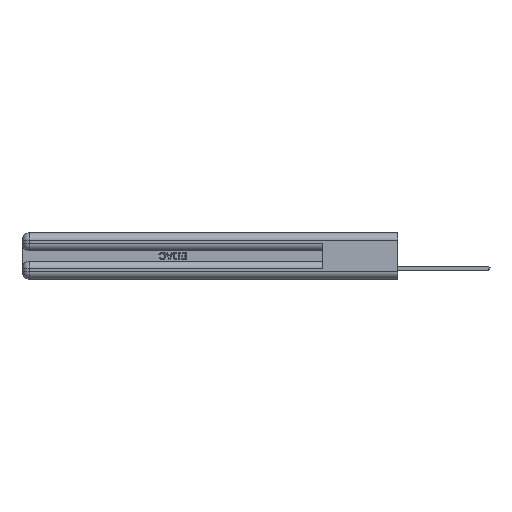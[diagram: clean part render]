
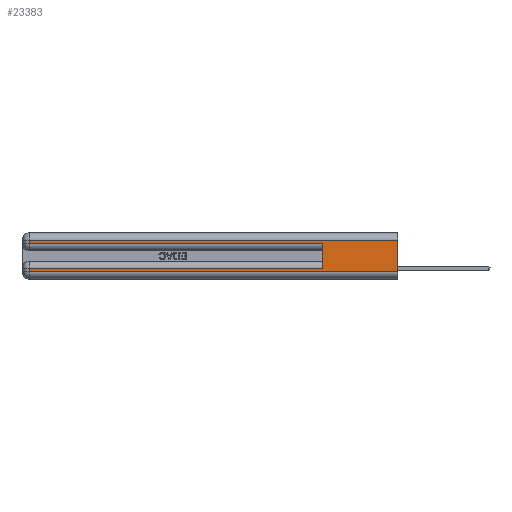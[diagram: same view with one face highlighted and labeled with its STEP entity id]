
A CAD part, left-side view. The second image highlights one B-rep face of the part: STEP entity #23383.
In plain terms, the highlighted planar face has unit normal (-1, 0, 0).
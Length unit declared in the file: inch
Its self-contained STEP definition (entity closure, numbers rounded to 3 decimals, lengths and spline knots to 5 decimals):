
#30 = EDGE_CURVE ( 'NONE', #2019, #31257, #36650, .T. ) ;
#2019 = VERTEX_POINT ( 'NONE', #28141 ) ;
#2697 = CARTESIAN_POINT ( 'NONE',  ( 0., 2.94, 0.37 ) ) ;
#3046 = VERTEX_POINT ( 'NONE', #7560 ) ;
#3961 = LINE ( 'NONE', #32662, #34732 ) ;
#4749 = ORIENTED_EDGE ( 'NONE', *, *, #12895, .T. ) ;
#5419 = DIRECTION ( 'NONE',  ( 0., 1., 0. ) ) ;
#5874 = ORIENTED_EDGE ( 'NONE', *, *, #6137, .T. ) ;
#6137 = EDGE_CURVE ( 'NONE', #37781, #32325, #39970, .T. ) ;
#6320 = DIRECTION ( 'NONE',  ( 0., 0., -1. ) ) ;
#6429 = CARTESIAN_POINT ( 'NONE',  ( 0., 2.94, 0.31 ) ) ;
#6513 = DIRECTION ( 'NONE',  ( 0., 0., -1. ) ) ;
#7024 = DIRECTION ( 'NONE',  ( 0., -1., 0. ) ) ;
#7560 = CARTESIAN_POINT ( 'NONE',  ( 0., 0., 0.06 ) ) ;
#8709 = CARTESIAN_POINT ( 'NONE',  ( 0., 2.94, 0.37 ) ) ;
#9394 = DIRECTION ( 'NONE',  ( 0., 0., -1. ) ) ;
#10166 = DIRECTION ( 'NONE',  ( 0., 0., -1. ) ) ;
#10271 = VECTOR ( 'NONE', #23456, 39.37008 ) ;
#12156 = DIRECTION ( 'NONE',  ( 0., 0., 1. ) ) ;
#12380 = VERTEX_POINT ( 'NONE', #21497 ) ;
#12895 = EDGE_CURVE ( 'NONE', #20216, #31358, #40212, .T. ) ;
#13265 = VECTOR ( 'NONE', #31248, 39.37008 ) ;
#15003 = FACE_OUTER_BOUND ( 'NONE', #32805, .T. ) ;
#17899 = EDGE_CURVE ( 'NONE', #32325, #31257, #18100, .T. ) ;
#18100 = LINE ( 'NONE', #27805, #13265 ) ;
#18894 = ORIENTED_EDGE ( 'NONE', *, *, #30, .F. ) ;
#20216 = VERTEX_POINT ( 'NONE', #31986 ) ;
#20361 = LINE ( 'NONE', #45865, #10271 ) ;
#21497 = CARTESIAN_POINT ( 'NONE',  ( 0., 0., 0.31 ) ) ;
#21922 = VECTOR ( 'NONE', #12156, 39.37008 ) ;
#22559 = VECTOR ( 'NONE', #6513, 39.37008 ) ;
#22879 = CARTESIAN_POINT ( 'NONE',  ( 0., 0.6, 0.145 ) ) ;
#23084 = ORIENTED_EDGE ( 'NONE', *, *, #17899, .T. ) ;
#23284 = LINE ( 'NONE', #36455, #32134 ) ;
#23383 = ADVANCED_FACE ( 'NONE', ( #15003 ), #35766, .F. ) ;
#23456 = DIRECTION ( 'NONE',  ( 0., 1., 0. ) ) ;
#27660 = VECTOR ( 'NONE', #5419, 39.37008 ) ;
#27805 = CARTESIAN_POINT ( 'NONE',  ( 0., 0., 0.285 ) ) ;
#28141 = CARTESIAN_POINT ( 'NONE',  ( 0., 0.6, 0.085 ) ) ;
#28303 = CARTESIAN_POINT ( 'NONE',  ( 0., 0., 0.37 ) ) ;
#28449 = CARTESIAN_POINT ( 'NONE',  ( 0., 0.6, 0.285 ) ) ;
#29963 = VECTOR ( 'NONE', #9394, 39.37008 ) ;
#30711 = ORIENTED_EDGE ( 'NONE', *, *, #32608, .T. ) ;
#31248 = DIRECTION ( 'NONE',  ( 0., -1., 0. ) ) ;
#31257 = VERTEX_POINT ( 'NONE', #28449 ) ;
#31358 = VERTEX_POINT ( 'NONE', #41608 ) ;
#31986 = CARTESIAN_POINT ( 'NONE',  ( 0., 2.94, 0.085 ) ) ;
#32134 = VECTOR ( 'NONE', #7024, 39.37008 ) ;
#32325 = VERTEX_POINT ( 'NONE', #40788 ) ;
#32608 = EDGE_CURVE ( 'NONE', #31358, #3046, #23284, .T. ) ;
#32662 = CARTESIAN_POINT ( 'NONE',  ( 0., 0., 0.37 ) ) ;
#32805 = EDGE_LOOP ( 'NONE', ( #47967, #44596, #5874, #23084, #18894, #33005, #4749, #30711 ) ) ;
#33005 = ORIENTED_EDGE ( 'NONE', *, *, #40183, .T. ) ;
#33127 = DIRECTION ( 'NONE',  ( 1., 0., 0. ) ) ;
#34732 = VECTOR ( 'NONE', #10166, 39.37008 ) ;
#35766 = PLANE ( 'NONE',  #40867 ) ;
#36455 = CARTESIAN_POINT ( 'NONE',  ( 0., 0., 0.06 ) ) ;
#36650 = LINE ( 'NONE', #22879, #21922 ) ;
#36848 = EDGE_CURVE ( 'NONE', #12380, #37781, #43692, .T. ) ;
#37781 = VERTEX_POINT ( 'NONE', #6429 ) ;
#38158 = EDGE_CURVE ( 'NONE', #12380, #3046, #3961, .T. ) ;
#39970 = LINE ( 'NONE', #8709, #29963 ) ;
#40183 = EDGE_CURVE ( 'NONE', #2019, #20216, #20361, .T. ) ;
#40212 = LINE ( 'NONE', #2697, #22559 ) ;
#40788 = CARTESIAN_POINT ( 'NONE',  ( 0., 2.94, 0.285 ) ) ;
#40867 = AXIS2_PLACEMENT_3D ( 'NONE', #28303, #33127, #6320 ) ;
#41608 = CARTESIAN_POINT ( 'NONE',  ( 0., 2.94, 0.06 ) ) ;
#43692 = LINE ( 'NONE', #46215, #27660 ) ;
#44596 = ORIENTED_EDGE ( 'NONE', *, *, #36848, .T. ) ;
#45865 = CARTESIAN_POINT ( 'NONE',  ( 0., 0., 0.085 ) ) ;
#46215 = CARTESIAN_POINT ( 'NONE',  ( 0., 0., 0.31 ) ) ;
#47967 = ORIENTED_EDGE ( 'NONE', *, *, #38158, .F. ) ;
